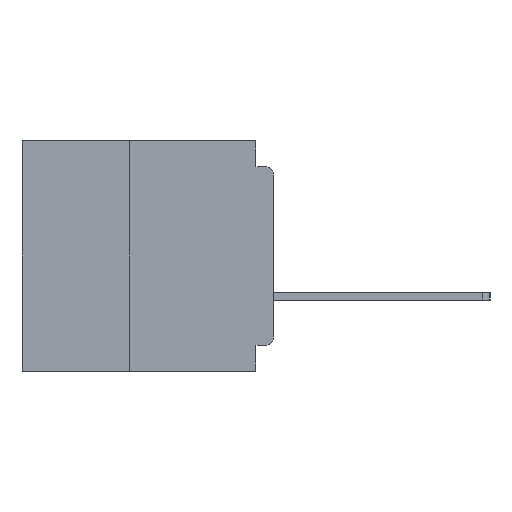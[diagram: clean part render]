
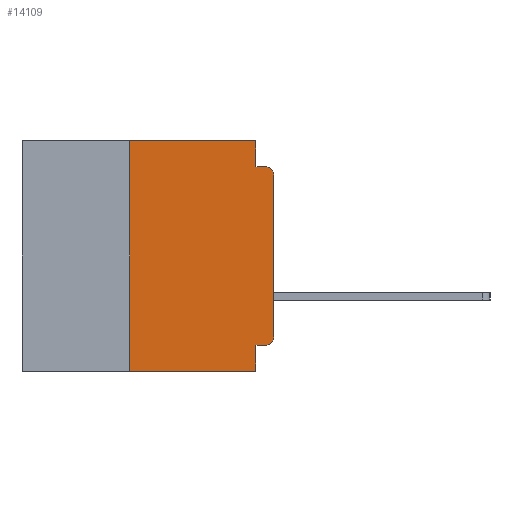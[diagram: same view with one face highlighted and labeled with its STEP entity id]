
A CAD part, left-side view. The second image highlights one B-rep face of the part: STEP entity #14109.
In plain terms, the highlighted planar face has unit normal (-1, 0, 0).
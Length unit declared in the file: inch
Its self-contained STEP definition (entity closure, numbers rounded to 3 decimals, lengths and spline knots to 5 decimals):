
#387 = CIRCLE ( 'NONE', #29974, 0.015 ) ;
#830 = VERTEX_POINT ( 'NONE', #36357 ) ;
#931 = DIRECTION ( 'NONE',  ( -1., 0., 0. ) ) ;
#1468 = AXIS2_PLACEMENT_3D ( 'NONE', #23136, #931, #26845 ) ;
#2143 = LINE ( 'NONE', #2186, #30541 ) ;
#2186 = CARTESIAN_POINT ( 'NONE',  ( 0., 0.437, 0. ) ) ;
#2659 = EDGE_CURVE ( 'NONE', #9871, #24899, #12381, .T. ) ;
#3863 = LINE ( 'NONE', #34936, #40774 ) ;
#5571 = ORIENTED_EDGE ( 'NONE', *, *, #16575, .F. ) ;
#5658 = CARTESIAN_POINT ( 'NONE',  ( 0., 0., -0.06 ) ) ;
#5931 = DIRECTION ( 'NONE',  ( 0., -1., 0. ) ) ;
#6119 = FACE_OUTER_BOUND ( 'NONE', #39122, .T. ) ;
#6190 = ORIENTED_EDGE ( 'NONE', *, *, #29648, .F. ) ;
#6284 = CARTESIAN_POINT ( 'NONE',  ( 0., 0.031, 0. ) ) ;
#6625 = CARTESIAN_POINT ( 'NONE',  ( 0., 0.25, 0. ) ) ;
#7414 = ORIENTED_EDGE ( 'NONE', *, *, #2659, .F. ) ;
#8775 = ORIENTED_EDGE ( 'NONE', *, *, #26435, .F. ) ;
#9463 = VERTEX_POINT ( 'NONE', #25683 ) ;
#9871 = VERTEX_POINT ( 'NONE', #24849 ) ;
#10134 = DIRECTION ( 'NONE',  ( 0., 0., -1. ) ) ;
#10588 = DIRECTION ( 'NONE',  ( -1., 0., 0. ) ) ;
#11796 = CARTESIAN_POINT ( 'NONE',  ( 0., 0., -0.34 ) ) ;
#12381 = LINE ( 'NONE', #26982, #35437 ) ;
#12911 = EDGE_CURVE ( 'NONE', #830, #31434, #22447, .T. ) ;
#12968 = EDGE_CURVE ( 'NONE', #35552, #29314, #387, .T. ) ;
#13548 = VECTOR ( 'NONE', #45819, 39.37008 ) ;
#14109 = ADVANCED_FACE ( 'NONE', ( #6119 ), #26467, .F. ) ;
#15482 = VECTOR ( 'NONE', #16576, 39.37008 ) ;
#16575 = EDGE_CURVE ( 'NONE', #24899, #830, #2143, .T. ) ;
#16576 = DIRECTION ( 'NONE',  ( 0., -1., 0. ) ) ;
#17772 = VERTEX_POINT ( 'NONE', #5658 ) ;
#18487 = VECTOR ( 'NONE', #10134, 39.37008 ) ;
#18815 = EDGE_CURVE ( 'NONE', #29314, #17772, #33170, .T. ) ;
#20145 = CARTESIAN_POINT ( 'NONE',  ( 0., 0., 0. ) ) ;
#21249 = VERTEX_POINT ( 'NONE', #24160 ) ;
#22214 = DIRECTION ( 'NONE',  ( 0., 0., 1. ) ) ;
#22447 = LINE ( 'NONE', #6284, #44264 ) ;
#22837 = ORIENTED_EDGE ( 'NONE', *, *, #12911, .F. ) ;
#22918 = DIRECTION ( 'NONE',  ( 0., 0., -1. ) ) ;
#23136 = CARTESIAN_POINT ( 'NONE',  ( 0., 0.015, -0.06 ) ) ;
#23788 = CARTESIAN_POINT ( 'NONE',  ( 0., 0., -0.045 ) ) ;
#24160 = CARTESIAN_POINT ( 'NONE',  ( 0., 0.015, -0.045 ) ) ;
#24383 = CARTESIAN_POINT ( 'NONE',  ( 0., 0.031, -0.045 ) ) ;
#24849 = CARTESIAN_POINT ( 'NONE',  ( 0., 0.25, -0.4 ) ) ;
#24899 = VERTEX_POINT ( 'NONE', #6625 ) ;
#25683 = CARTESIAN_POINT ( 'NONE',  ( 0., 0.031, -0.355 ) ) ;
#26435 = EDGE_CURVE ( 'NONE', #31434, #21249, #44783, .T. ) ;
#26467 = PLANE ( 'NONE',  #36166 ) ;
#26845 = DIRECTION ( 'NONE',  ( 0., 0., -1. ) ) ;
#26882 = ORIENTED_EDGE ( 'NONE', *, *, #35603, .T. ) ;
#26982 = CARTESIAN_POINT ( 'NONE',  ( 0., 0.25, -0.4 ) ) ;
#27136 = LINE ( 'NONE', #35901, #18487 ) ;
#27507 = CARTESIAN_POINT ( 'NONE',  ( 0., 0.031, -0.4 ) ) ;
#27514 = DIRECTION ( 'NONE',  ( 0., -1., 0. ) ) ;
#27791 = LINE ( 'NONE', #39118, #46123 ) ;
#28535 = CIRCLE ( 'NONE', #1468, 0.015 ) ;
#28970 = ORIENTED_EDGE ( 'NONE', *, *, #18815, .T. ) ;
#29000 = EDGE_CURVE ( 'NONE', #35552, #9463, #27791, .T. ) ;
#29314 = VERTEX_POINT ( 'NONE', #11796 ) ;
#29648 = EDGE_CURVE ( 'NONE', #9463, #36540, #27136, .T. ) ;
#29974 = AXIS2_PLACEMENT_3D ( 'NONE', #32682, #10588, #36336 ) ;
#30190 = CARTESIAN_POINT ( 'NONE',  ( 0., 0.437, 0. ) ) ;
#30382 = ORIENTED_EDGE ( 'NONE', *, *, #29000, .F. ) ;
#30541 = VECTOR ( 'NONE', #5931, 39.37008 ) ;
#31434 = VERTEX_POINT ( 'NONE', #24383 ) ;
#31660 = DIRECTION ( 'NONE',  ( 0., 1., 0. ) ) ;
#32682 = CARTESIAN_POINT ( 'NONE',  ( 0., 0.015, -0.34 ) ) ;
#33002 = CARTESIAN_POINT ( 'NONE',  ( 0., 0.015, -0.355 ) ) ;
#33170 = LINE ( 'NONE', #20145, #13548 ) ;
#34936 = CARTESIAN_POINT ( 'NONE',  ( 0., 0.437, -0.4 ) ) ;
#35437 = VECTOR ( 'NONE', #22214, 39.37008 ) ;
#35552 = VERTEX_POINT ( 'NONE', #33002 ) ;
#35603 = EDGE_CURVE ( 'NONE', #17772, #21249, #28535, .T. ) ;
#35901 = CARTESIAN_POINT ( 'NONE',  ( 0., 0.031, -0.4 ) ) ;
#36166 = AXIS2_PLACEMENT_3D ( 'NONE', #30190, #44900, #22918 ) ;
#36336 = DIRECTION ( 'NONE',  ( 0., 0., -1. ) ) ;
#36357 = CARTESIAN_POINT ( 'NONE',  ( 0., 0.031, 0. ) ) ;
#36540 = VERTEX_POINT ( 'NONE', #27507 ) ;
#38717 = ORIENTED_EDGE ( 'NONE', *, *, #47781, .T. ) ;
#39118 = CARTESIAN_POINT ( 'NONE',  ( 0., 0., -0.355 ) ) ;
#39122 = EDGE_LOOP ( 'NONE', ( #28970, #26882, #8775, #22837, #5571, #7414, #38717, #6190, #30382, #45848 ) ) ;
#40774 = VECTOR ( 'NONE', #27514, 39.37008 ) ;
#43151 = DIRECTION ( 'NONE',  ( 0., 0., -1. ) ) ;
#44264 = VECTOR ( 'NONE', #43151, 39.37008 ) ;
#44783 = LINE ( 'NONE', #23788, #15482 ) ;
#44900 = DIRECTION ( 'NONE',  ( 1., 0., 0. ) ) ;
#45819 = DIRECTION ( 'NONE',  ( 0., 0., 1. ) ) ;
#45848 = ORIENTED_EDGE ( 'NONE', *, *, #12968, .T. ) ;
#46123 = VECTOR ( 'NONE', #31660, 39.37008 ) ;
#47781 = EDGE_CURVE ( 'NONE', #9871, #36540, #3863, .T. ) ;
